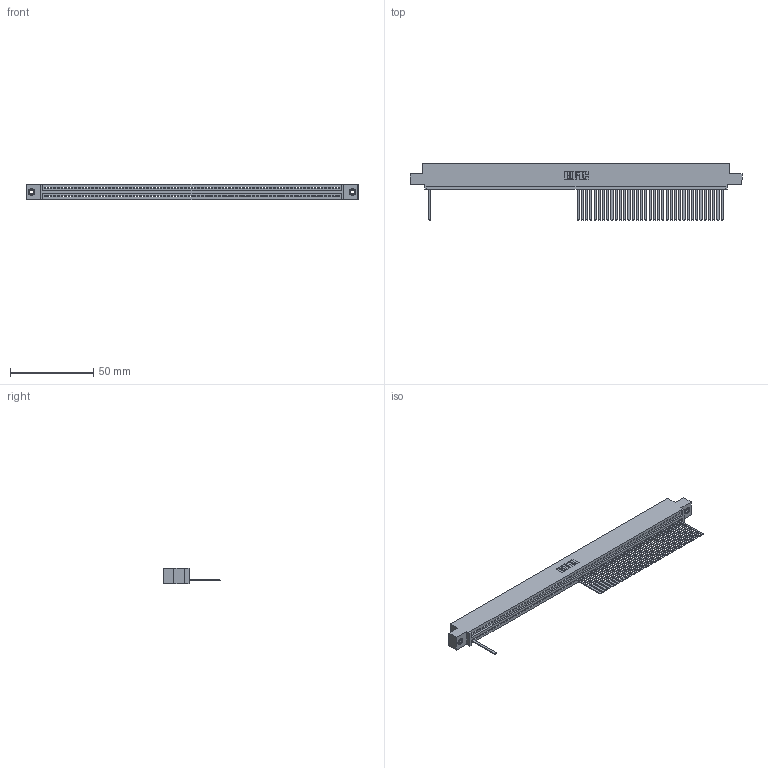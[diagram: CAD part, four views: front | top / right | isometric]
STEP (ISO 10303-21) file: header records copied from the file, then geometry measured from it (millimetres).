
FILE_DESCRIPTION (( 'STEP AP203' ), '1' );
FILE_NAME ('395-070-544-408.STEP', '2018-11-26T23:08:36', ( '' ), ( '' ), 'SwSTEP 2.0', 'SolidWorks 2016', '' );
FILE_SCHEMA (( 'CONFIG_CONTROL_DESIGN' ));
Length unit declared in the file: inch
Products named in the file (4): 395-070-544-408; 345-292-001_345-293-144; 345-250-001_345-250-003-102; 345 Part_0.110 Offset - 0.156 Dia-TI
Assembly tree (39 placements, depth 2):
  395-070-544-408
    345 Part_0.110 Offset - 0.156 Dia-TI
    345-292-001_345-293-144  x36
    345-250-001_345-250-003-102  x2
Bounding box: 199.01 x 33.96 x 9.4 mm (x, y, z)
Volume: 19079.2 mm3; surface area: 25020.2 mm2
Topology: 39 solids, 39 shells, 2606 faces, 8013 edges, 5286 vertices
Faces by surface type: plane 1888, cylinder 702, cone 12, torus 4
Entity records: 48960 total; most frequent: ORIENTED_EDGE 8646, CARTESIAN_POINT 8615, DIRECTION 7469, EDGE_CURVE 4323, LINE 3895, VECTOR 3895, VERTEX_POINT 2876, AXIS2_PLACEMENT_3D 1787
